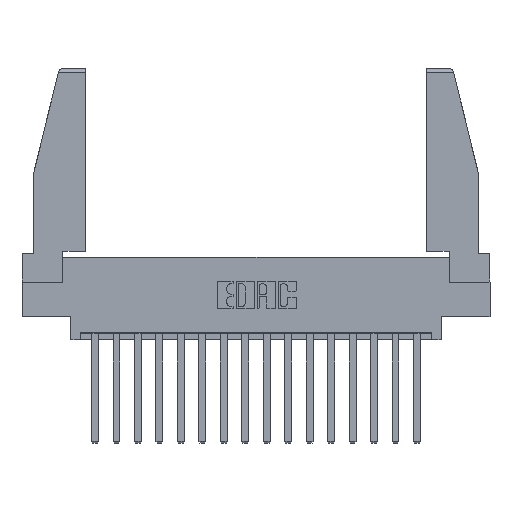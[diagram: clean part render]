
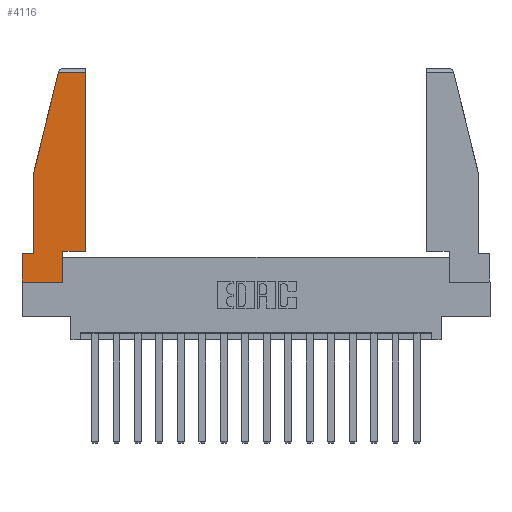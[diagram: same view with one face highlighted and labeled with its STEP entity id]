
A CAD part, top view. The second image highlights one B-rep face of the part: STEP entity #4116.
In plain terms, the highlighted planar face has unit normal (0, 0, 1).
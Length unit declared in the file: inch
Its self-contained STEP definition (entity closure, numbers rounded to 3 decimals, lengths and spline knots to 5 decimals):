
#92 = LINE ( 'NONE', #452, #2499 ) ;
#425 = ORIENTED_EDGE ( 'NONE', *, *, #12630, .T. ) ;
#452 = CARTESIAN_POINT ( 'NONE',  ( 0.086, 0.8, 0. ) ) ;
#576 = CARTESIAN_POINT ( 'NONE',  ( 0., 0., 0. ) ) ;
#638 = LINE ( 'NONE', #12675, #3907 ) ;
#1065 = DIRECTION ( 'NONE',  ( 0., 1., 0. ) ) ;
#1097 = CARTESIAN_POINT ( 'NONE',  ( 0., 0.21, 0. ) ) ;
#1610 = EDGE_CURVE ( 'NONE', #16601, #14931, #16024, .T. ) ;
#1876 = DIRECTION ( 'NONE',  ( 0., -1., 0. ) ) ;
#2090 = EDGE_CURVE ( 'NONE', #12069, #16838, #15324, .T. ) ;
#2499 = VECTOR ( 'NONE', #1876, 39.37008 ) ;
#3083 = VERTEX_POINT ( 'NONE', #9501 ) ;
#3134 = CARTESIAN_POINT ( 'NONE',  ( 0.271, 1.55, 0. ) ) ;
#3304 = CARTESIAN_POINT ( 'NONE',  ( 0.461, 0.223, 0. ) ) ;
#3772 = VECTOR ( 'NONE', #15812, 39.37008 ) ;
#3891 = CARTESIAN_POINT ( 'NONE',  ( 0.297, 0.223, 0. ) ) ;
#3907 = VECTOR ( 'NONE', #11216, 39.37008 ) ;
#4116 = ADVANCED_FACE ( 'NONE', ( #9513 ), #12944, .T. ) ;
#4171 = LINE ( 'NONE', #12858, #6874 ) ;
#4628 = LINE ( 'NONE', #5461, #8818 ) ;
#4634 = VECTOR ( 'NONE', #6486, 39.37008 ) ;
#5443 = LINE ( 'NONE', #10852, #12002 ) ;
#5461 = CARTESIAN_POINT ( 'NONE',  ( 0., 0.21, 0. ) ) ;
#5528 = DIRECTION ( 'NONE',  ( -1., 0., 0. ) ) ;
#5742 = CARTESIAN_POINT ( 'NONE',  ( 0.297, 0., 0. ) ) ;
#6124 = DIRECTION ( 'NONE',  ( 0., 0., 1. ) ) ;
#6486 = DIRECTION ( 'NONE',  ( 0., 1., 0. ) ) ;
#6629 = DIRECTION ( 'NONE',  ( 0., -1., 0. ) ) ;
#6850 = VERTEX_POINT ( 'NONE', #8436 ) ;
#6874 = VECTOR ( 'NONE', #11641, 39.37008 ) ;
#7101 = CARTESIAN_POINT ( 'NONE',  ( 0.086, 0.21, 0. ) ) ;
#7840 = VERTEX_POINT ( 'NONE', #10509 ) ;
#8068 = VERTEX_POINT ( 'NONE', #7101 ) ;
#8389 = LINE ( 'NONE', #10670, #4634 ) ;
#8436 = CARTESIAN_POINT ( 'NONE',  ( 0.461, 1.52, 0. ) ) ;
#8546 = EDGE_CURVE ( 'NONE', #8068, #12069, #4628, .T. ) ;
#8818 = VECTOR ( 'NONE', #5528, 39.37008 ) ;
#9057 = EDGE_CURVE ( 'NONE', #6850, #3083, #4171, .T. ) ;
#9136 = VERTEX_POINT ( 'NONE', #3304 ) ;
#9229 = ORIENTED_EDGE ( 'NONE', *, *, #10582, .T. ) ;
#9501 = CARTESIAN_POINT ( 'NONE',  ( 0.2636, 1.52, 0. ) ) ;
#9513 = FACE_OUTER_BOUND ( 'NONE', #16871, .T. ) ;
#9708 = LINE ( 'NONE', #3134, #3772 ) ;
#10509 = CARTESIAN_POINT ( 'NONE',  ( 0.086, 0.8, 0. ) ) ;
#10582 = EDGE_CURVE ( 'NONE', #14931, #9136, #5443, .T. ) ;
#10628 = ORIENTED_EDGE ( 'NONE', *, *, #14120, .T. ) ;
#10670 = CARTESIAN_POINT ( 'NONE',  ( 0.461, 0.223, 0. ) ) ;
#10852 = CARTESIAN_POINT ( 'NONE',  ( 0.297, 0.223, 0. ) ) ;
#11216 = DIRECTION ( 'NONE',  ( 1., 0., 0. ) ) ;
#11641 = DIRECTION ( 'NONE',  ( -1., 0., 0. ) ) ;
#12002 = VECTOR ( 'NONE', #15237, 39.37008 ) ;
#12029 = AXIS2_PLACEMENT_3D ( 'NONE', #13178, #6124, #16079 ) ;
#12069 = VERTEX_POINT ( 'NONE', #12312 ) ;
#12312 = CARTESIAN_POINT ( 'NONE',  ( 0., 0.21, 0. ) ) ;
#12497 = ORIENTED_EDGE ( 'NONE', *, *, #8546, .T. ) ;
#12630 = EDGE_CURVE ( 'NONE', #7840, #8068, #92, .T. ) ;
#12675 = CARTESIAN_POINT ( 'NONE',  ( 0., 0., 0. ) ) ;
#12858 = CARTESIAN_POINT ( 'NONE',  ( 0., 1.52, 0. ) ) ;
#12944 = PLANE ( 'NONE',  #12029 ) ;
#13178 = CARTESIAN_POINT ( 'NONE',  ( 0., 0., 0. ) ) ;
#13873 = EDGE_CURVE ( 'NONE', #3083, #7840, #9708, .T. ) ;
#14120 = EDGE_CURVE ( 'NONE', #9136, #6850, #8389, .T. ) ;
#14657 = ORIENTED_EDGE ( 'NONE', *, *, #16046, .T. ) ;
#14931 = VERTEX_POINT ( 'NONE', #3891 ) ;
#15038 = ORIENTED_EDGE ( 'NONE', *, *, #1610, .T. ) ;
#15237 = DIRECTION ( 'NONE',  ( 1., 0., 0. ) ) ;
#15284 = CARTESIAN_POINT ( 'NONE',  ( 0.297, 0., 0. ) ) ;
#15324 = LINE ( 'NONE', #1097, #18169 ) ;
#15381 = ORIENTED_EDGE ( 'NONE', *, *, #13873, .T. ) ;
#15812 = DIRECTION ( 'NONE',  ( -0.239, -0.971, 0. ) ) ;
#16024 = LINE ( 'NONE', #15284, #17338 ) ;
#16046 = EDGE_CURVE ( 'NONE', #16838, #16601, #638, .T. ) ;
#16079 = DIRECTION ( 'NONE',  ( 1., 0., 0. ) ) ;
#16489 = ORIENTED_EDGE ( 'NONE', *, *, #2090, .T. ) ;
#16601 = VERTEX_POINT ( 'NONE', #5742 ) ;
#16838 = VERTEX_POINT ( 'NONE', #576 ) ;
#16871 = EDGE_LOOP ( 'NONE', ( #10628, #17600, #15381, #425, #12497, #16489, #14657, #15038, #9229 ) ) ;
#17338 = VECTOR ( 'NONE', #1065, 39.37008 ) ;
#17600 = ORIENTED_EDGE ( 'NONE', *, *, #9057, .T. ) ;
#18169 = VECTOR ( 'NONE', #6629, 39.37008 ) ;
